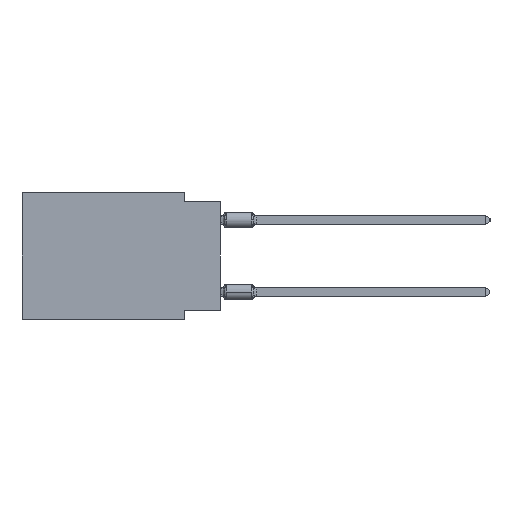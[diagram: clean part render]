
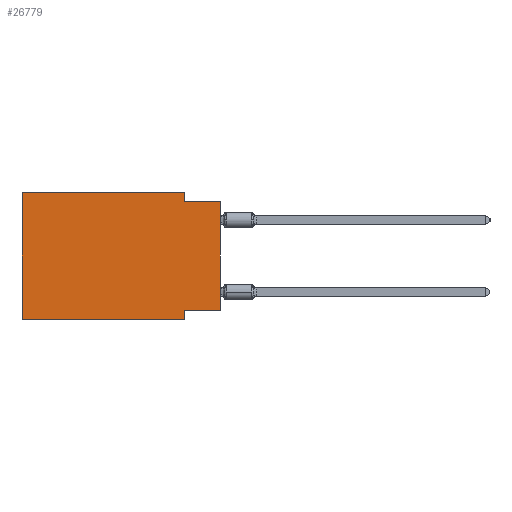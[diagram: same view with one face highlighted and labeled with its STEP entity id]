
A CAD part, left-side view. The second image highlights one B-rep face of the part: STEP entity #26779.
In plain terms, the highlighted planar face has unit normal (-1, 0, 0).
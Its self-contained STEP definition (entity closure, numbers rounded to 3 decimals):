
#167 = VECTOR ( 'NONE', #18843, 1000. ) ;
#822 = LINE ( 'NONE', #22233, #18280 ) ;
#959 = CARTESIAN_POINT ( 'NONE',  ( 0., 2.54, 0. ) ) ;
#2401 = FACE_OUTER_BOUND ( 'NONE', #27375, .T. ) ;
#4469 = VECTOR ( 'NONE', #28829, 1000. ) ;
#4855 = VECTOR ( 'NONE', #22975, 1000. ) ;
#5330 = ORIENTED_EDGE ( 'NONE', *, *, #25934, .T. ) ;
#5464 = DIRECTION ( 'NONE',  ( 0., 0., 1. ) ) ;
#6425 = EDGE_CURVE ( 'NONE', #13787, #21457, #27282, .T. ) ;
#8018 = LINE ( 'NONE', #20015, #35217 ) ;
#8375 = LINE ( 'NONE', #29411, #33719 ) ;
#8422 = CARTESIAN_POINT ( 'NONE',  ( 0., 13.97, 0. ) ) ;
#9251 = ORIENTED_EDGE ( 'NONE', *, *, #31733, .F. ) ;
#9697 = ORIENTED_EDGE ( 'NONE', *, *, #22185, .F. ) ;
#10346 = CARTESIAN_POINT ( 'NONE',  ( 0., 13.97, 0. ) ) ;
#10854 = DIRECTION ( 'NONE',  ( 0., 0., -1. ) ) ;
#10918 = CARTESIAN_POINT ( 'NONE',  ( 0., 2.54, -8.89 ) ) ;
#11128 = LINE ( 'NONE', #10346, #4469 ) ;
#11134 = EDGE_CURVE ( 'NONE', #16473, #20675, #822, .T. ) ;
#11191 = CARTESIAN_POINT ( 'NONE',  ( 0., 13.97, -8.89 ) ) ;
#12590 = ORIENTED_EDGE ( 'NONE', *, *, #33267, .F. ) ;
#13523 = ORIENTED_EDGE ( 'NONE', *, *, #11134, .T. ) ;
#13787 = VERTEX_POINT ( 'NONE', #959 ) ;
#13892 = EDGE_CURVE ( 'NONE', #21457, #20675, #8375, .T. ) ;
#13942 = CARTESIAN_POINT ( 'NONE',  ( 0., 0., -0.635 ) ) ;
#13979 = VERTEX_POINT ( 'NONE', #20939 ) ;
#16473 = VERTEX_POINT ( 'NONE', #26916 ) ;
#16864 = AXIS2_PLACEMENT_3D ( 'NONE', #37966, #22835, #10854 ) ;
#17027 = DIRECTION ( 'NONE',  ( 0., -1., 0. ) ) ;
#17488 = ORIENTED_EDGE ( 'NONE', *, *, #34376, .F. ) ;
#18280 = VECTOR ( 'NONE', #20077, 1000. ) ;
#18843 = DIRECTION ( 'NONE',  ( 0., 0., -1. ) ) ;
#19672 = ORIENTED_EDGE ( 'NONE', *, *, #13892, .F. ) ;
#19798 = CARTESIAN_POINT ( 'NONE',  ( 0., 2.54, -8.89 ) ) ;
#19969 = DIRECTION ( 'NONE',  ( 0., 0., -1. ) ) ;
#20015 = CARTESIAN_POINT ( 'NONE',  ( 0., 0., -8.255 ) ) ;
#20077 = DIRECTION ( 'NONE',  ( 0., 0., 1. ) ) ;
#20621 = VECTOR ( 'NONE', #19969, 1000. ) ;
#20675 = VERTEX_POINT ( 'NONE', #13942 ) ;
#20939 = CARTESIAN_POINT ( 'NONE',  ( 0., 2.54, -8.255 ) ) ;
#21457 = VERTEX_POINT ( 'NONE', #34835 ) ;
#21586 = CARTESIAN_POINT ( 'NONE',  ( 0., 2.54, 0. ) ) ;
#22185 = EDGE_CURVE ( 'NONE', #32142, #13787, #11128, .T. ) ;
#22233 = CARTESIAN_POINT ( 'NONE',  ( 0., 0., 0. ) ) ;
#22835 = DIRECTION ( 'NONE',  ( 1., 0., 0. ) ) ;
#22975 = DIRECTION ( 'NONE',  ( 0., -1., 0. ) ) ;
#25934 = EDGE_CURVE ( 'NONE', #29248, #35894, #29480, .T. ) ;
#26076 = ORIENTED_EDGE ( 'NONE', *, *, #6425, .F. ) ;
#26312 = VECTOR ( 'NONE', #5464, 1000. ) ;
#26749 = PLANE ( 'NONE',  #16864 ) ;
#26779 = ADVANCED_FACE ( 'NONE', ( #2401 ), #26749, .F. ) ;
#26916 = CARTESIAN_POINT ( 'NONE',  ( 0., 0., -8.255 ) ) ;
#27282 = LINE ( 'NONE', #21586, #167 ) ;
#27375 = EDGE_LOOP ( 'NONE', ( #13523, #19672, #26076, #9697, #17488, #5330, #12590, #9251 ) ) ;
#28829 = DIRECTION ( 'NONE',  ( 0., -1., 0. ) ) ;
#29248 = VERTEX_POINT ( 'NONE', #32913 ) ;
#29411 = CARTESIAN_POINT ( 'NONE',  ( 0., 0., -0.635 ) ) ;
#29480 = LINE ( 'NONE', #11191, #4855 ) ;
#31029 = LINE ( 'NONE', #10918, #20621 ) ;
#31733 = EDGE_CURVE ( 'NONE', #16473, #13979, #8018, .T. ) ;
#32000 = DIRECTION ( 'NONE',  ( 0., 1., 0. ) ) ;
#32142 = VERTEX_POINT ( 'NONE', #32911 ) ;
#32911 = CARTESIAN_POINT ( 'NONE',  ( 0., 13.97, 0. ) ) ;
#32913 = CARTESIAN_POINT ( 'NONE',  ( 0., 13.97, -8.89 ) ) ;
#33267 = EDGE_CURVE ( 'NONE', #13979, #35894, #31029, .T. ) ;
#33719 = VECTOR ( 'NONE', #17027, 1000. ) ;
#34376 = EDGE_CURVE ( 'NONE', #29248, #32142, #35340, .T. ) ;
#34835 = CARTESIAN_POINT ( 'NONE',  ( 0., 2.54, -0.635 ) ) ;
#35217 = VECTOR ( 'NONE', #32000, 1000. ) ;
#35340 = LINE ( 'NONE', #8422, #26312 ) ;
#35894 = VERTEX_POINT ( 'NONE', #19798 ) ;
#37966 = CARTESIAN_POINT ( 'NONE',  ( 0., 13.97, 0. ) ) ;
